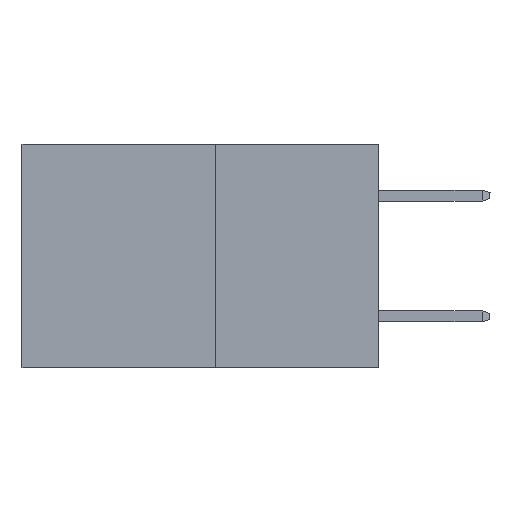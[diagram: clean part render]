
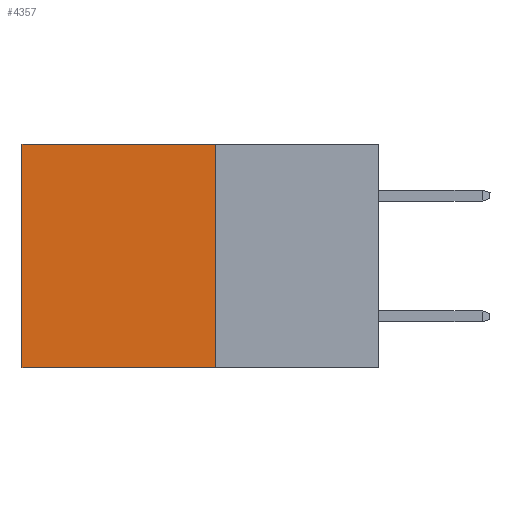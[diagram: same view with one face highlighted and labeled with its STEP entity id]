
A CAD part, left-side view. The second image highlights one B-rep face of the part: STEP entity #4357.
In plain terms, the highlighted planar face has unit normal (-1, 0, 0).
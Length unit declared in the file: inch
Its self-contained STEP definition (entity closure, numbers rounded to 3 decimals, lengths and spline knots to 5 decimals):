
#126 = EDGE_CURVE ( 'NONE', #7766, #7951, #5513, .T. ) ;
#514 = DIRECTION ( 'NONE',  ( 0., 0., -1. ) ) ;
#930 = DIRECTION ( 'NONE',  ( 0., 1., 0. ) ) ;
#1008 = CARTESIAN_POINT ( 'NONE',  ( 0.277, 0.27, 0. ) ) ;
#1037 = LINE ( 'NONE', #1228, #9438 ) ;
#1228 = CARTESIAN_POINT ( 'NONE',  ( 0.277, 0.59, -0.37 ) ) ;
#1928 = CARTESIAN_POINT ( 'NONE',  ( 0.277, 0.59, -0.37 ) ) ;
#2017 = DIRECTION ( 'NONE',  ( 1., 0., 0. ) ) ;
#2361 = DIRECTION ( 'NONE',  ( 0., 0., -1. ) ) ;
#2875 = CARTESIAN_POINT ( 'NONE',  ( 0.277, 0.27, -0.37 ) ) ;
#2879 = LINE ( 'NONE', #3260, #5204 ) ;
#3090 = ORIENTED_EDGE ( 'NONE', *, *, #11327, .T. ) ;
#3260 = CARTESIAN_POINT ( 'NONE',  ( 0.277, 0.27, 0. ) ) ;
#4333 = FACE_OUTER_BOUND ( 'NONE', #8538, .T. ) ;
#4357 = ADVANCED_FACE ( 'NONE', ( #4333 ), #8875, .F. ) ;
#4817 = VECTOR ( 'NONE', #514, 39.37008 ) ;
#4845 = ORIENTED_EDGE ( 'NONE', *, *, #126, .F. ) ;
#5160 = VERTEX_POINT ( 'NONE', #1008 ) ;
#5204 = VECTOR ( 'NONE', #930, 39.37008 ) ;
#5513 = LINE ( 'NONE', #2875, #8197 ) ;
#5923 = CARTESIAN_POINT ( 'NONE',  ( 0.277, 0.59, 0. ) ) ;
#6008 = ORIENTED_EDGE ( 'NONE', *, *, #6551, .T. ) ;
#6551 = EDGE_CURVE ( 'NONE', #5160, #7734, #2879, .T. ) ;
#7734 = VERTEX_POINT ( 'NONE', #5923 ) ;
#7766 = VERTEX_POINT ( 'NONE', #8284 ) ;
#7951 = VERTEX_POINT ( 'NONE', #1928 ) ;
#8197 = VECTOR ( 'NONE', #9734, 39.37008 ) ;
#8284 = CARTESIAN_POINT ( 'NONE',  ( 0.277, 0.27, -0.37 ) ) ;
#8538 = EDGE_LOOP ( 'NONE', ( #3090, #4845, #9884, #6008 ) ) ;
#8875 = PLANE ( 'NONE',  #10234 ) ;
#9438 = VECTOR ( 'NONE', #2361, 39.37008 ) ;
#9734 = DIRECTION ( 'NONE',  ( 0., 1., 0. ) ) ;
#9884 = ORIENTED_EDGE ( 'NONE', *, *, #13147, .F. ) ;
#10023 = DIRECTION ( 'NONE',  ( 0., 0., -1. ) ) ;
#10234 = AXIS2_PLACEMENT_3D ( 'NONE', #14565, #2017, #10023 ) ;
#10542 = LINE ( 'NONE', #10807, #4817 ) ;
#10807 = CARTESIAN_POINT ( 'NONE',  ( 0.277, 0.27, -0.37 ) ) ;
#11327 = EDGE_CURVE ( 'NONE', #7734, #7951, #1037, .T. ) ;
#13147 = EDGE_CURVE ( 'NONE', #5160, #7766, #10542, .T. ) ;
#14565 = CARTESIAN_POINT ( 'NONE',  ( 0.277, 0.27, -0.37 ) ) ;
